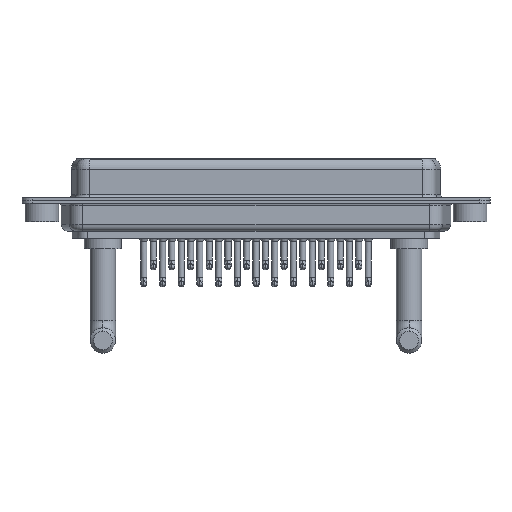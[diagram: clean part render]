
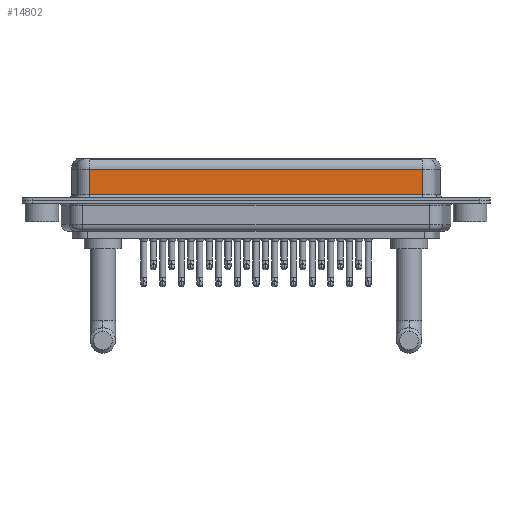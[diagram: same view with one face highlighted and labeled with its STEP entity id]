
A CAD part, front view. The second image highlights one B-rep face of the part: STEP entity #14802.
In plain terms, the highlighted planar face has unit normal (0, -1, 0).
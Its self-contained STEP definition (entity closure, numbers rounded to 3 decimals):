
#346 = FACE_OUTER_BOUND ( 'NONE', #22064, .T. ) ;
#978 = CARTESIAN_POINT ( 'NONE',  ( 56.462, -3.95, 4.65 ) ) ;
#992 = LINE ( 'NONE', #4757, #18746 ) ;
#1659 = DIRECTION ( 'NONE',  ( 0., 0., -1. ) ) ;
#2291 = AXIS2_PLACEMENT_3D ( 'NONE', #4229, #19532, #2360 ) ;
#2360 = DIRECTION ( 'NONE',  ( 0., 0., 1. ) ) ;
#3453 = EDGE_CURVE ( 'NONE', #6531, #4988, #8912, .T. ) ;
#4229 = CARTESIAN_POINT ( 'NONE',  ( 56.462, -3.95, 6.4 ) ) ;
#4360 = ORIENTED_EDGE ( 'NONE', *, *, #10047, .T. ) ;
#4757 = CARTESIAN_POINT ( 'NONE',  ( 56.462, -3.95, 4.65 ) ) ;
#4899 = VECTOR ( 'NONE', #1659, 1000. ) ;
#4988 = VERTEX_POINT ( 'NONE', #17228 ) ;
#5902 = DIRECTION ( 'NONE',  ( 0., 0., -1. ) ) ;
#6370 = LINE ( 'NONE', #20038, #6967 ) ;
#6472 = ORIENTED_EDGE ( 'NONE', *, *, #17311, .T. ) ;
#6531 = VERTEX_POINT ( 'NONE', #978 ) ;
#6581 = EDGE_CURVE ( 'NONE', #15884, #4988, #6370, .T. ) ;
#6789 = CARTESIAN_POINT ( 'NONE',  ( 7.038, -3.95, 0.9 ) ) ;
#6967 = VECTOR ( 'NONE', #14014, 1000. ) ;
#7978 = PLANE ( 'NONE',  #2291 ) ;
#8912 = LINE ( 'NONE', #24718, #4899 ) ;
#10047 = EDGE_CURVE ( 'NONE', #11193, #15884, #13191, .T. ) ;
#11193 = VERTEX_POINT ( 'NONE', #20296 ) ;
#13191 = LINE ( 'NONE', #22966, #17459 ) ;
#14014 = DIRECTION ( 'NONE',  ( 1., 0., 0. ) ) ;
#14274 = DIRECTION ( 'NONE',  ( -1., 0., 0. ) ) ;
#14802 = ADVANCED_FACE ( 'NONE', ( #346 ), #7978, .F. ) ;
#15884 = VERTEX_POINT ( 'NONE', #6789 ) ;
#16297 = ORIENTED_EDGE ( 'NONE', *, *, #6581, .T. ) ;
#17228 = CARTESIAN_POINT ( 'NONE',  ( 56.462, -3.95, 0.9 ) ) ;
#17311 = EDGE_CURVE ( 'NONE', #6531, #11193, #992, .T. ) ;
#17459 = VECTOR ( 'NONE', #5902, 1000. ) ;
#18610 = ORIENTED_EDGE ( 'NONE', *, *, #3453, .F. ) ;
#18746 = VECTOR ( 'NONE', #14274, 1000. ) ;
#19532 = DIRECTION ( 'NONE',  ( 0., 1., 0. ) ) ;
#20038 = CARTESIAN_POINT ( 'NONE',  ( 56.462, -3.95, 0.9 ) ) ;
#20296 = CARTESIAN_POINT ( 'NONE',  ( 7.038, -3.95, 4.65 ) ) ;
#22064 = EDGE_LOOP ( 'NONE', ( #18610, #6472, #4360, #16297 ) ) ;
#22966 = CARTESIAN_POINT ( 'NONE',  ( 7.038, -3.95, 6.4 ) ) ;
#24718 = CARTESIAN_POINT ( 'NONE',  ( 56.462, -3.95, 6.4 ) ) ;
